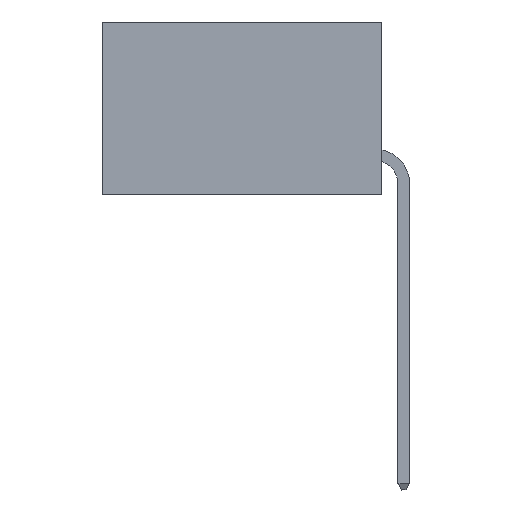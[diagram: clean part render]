
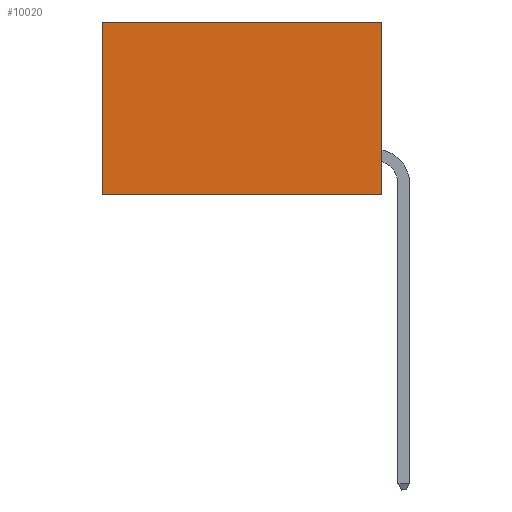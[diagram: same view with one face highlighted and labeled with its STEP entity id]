
A CAD part, left-side view. The second image highlights one B-rep face of the part: STEP entity #10020.
In plain terms, the highlighted planar face has unit normal (-1, 0, 0).
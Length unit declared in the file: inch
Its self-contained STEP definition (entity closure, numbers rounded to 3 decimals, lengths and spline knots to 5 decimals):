
#1034 = VECTOR ( 'NONE', #22122, 39.37008 ) ;
#3117 = DIRECTION ( 'NONE',  ( 1., 0., 0. ) ) ;
#3304 = DIRECTION ( 'NONE',  ( 0., 0., -1. ) ) ;
#5095 = CARTESIAN_POINT ( 'NONE',  ( 0.2875, 0., 0. ) ) ;
#5761 = EDGE_CURVE ( 'NONE', #21512, #16290, #15550, .T. ) ;
#6650 = FACE_OUTER_BOUND ( 'NONE', #12455, .T. ) ;
#6757 = AXIS2_PLACEMENT_3D ( 'NONE', #5095, #3117, #19487 ) ;
#6981 = CARTESIAN_POINT ( 'NONE',  ( 0.2875, 0., -0.37 ) ) ;
#7679 = ORIENTED_EDGE ( 'NONE', *, *, #8246, .F. ) ;
#8040 = CARTESIAN_POINT ( 'NONE',  ( 0.2875, 0., 0. ) ) ;
#8239 = PLANE ( 'NONE',  #6757 ) ;
#8246 = EDGE_CURVE ( 'NONE', #15647, #17259, #15751, .T. ) ;
#8665 = CARTESIAN_POINT ( 'NONE',  ( 0.2875, 0.6, 0. ) ) ;
#9180 = CARTESIAN_POINT ( 'NONE',  ( 0.2875, 0., 0. ) ) ;
#10020 = ADVANCED_FACE ( 'NONE', ( #6650 ), #8239, .F. ) ;
#11450 = ORIENTED_EDGE ( 'NONE', *, *, #15727, .F. ) ;
#11803 = VECTOR ( 'NONE', #3304, 39.37008 ) ;
#12327 = LINE ( 'NONE', #14745, #1034 ) ;
#12363 = VECTOR ( 'NONE', #17718, 39.37008 ) ;
#12455 = EDGE_LOOP ( 'NONE', ( #22738, #7679, #11450, #16863 ) ) ;
#12616 = LINE ( 'NONE', #19821, #11803 ) ;
#14745 = CARTESIAN_POINT ( 'NONE',  ( 0.2875, 0., 0. ) ) ;
#14821 = CARTESIAN_POINT ( 'NONE',  ( 0.2875, 0., -0.37 ) ) ;
#14979 = VECTOR ( 'NONE', #15838, 39.37008 ) ;
#15475 = EDGE_CURVE ( 'NONE', #16290, #17259, #12616, .T. ) ;
#15550 = LINE ( 'NONE', #8040, #14979 ) ;
#15647 = VERTEX_POINT ( 'NONE', #14821 ) ;
#15727 = EDGE_CURVE ( 'NONE', #21512, #15647, #12327, .T. ) ;
#15751 = LINE ( 'NONE', #6981, #12363 ) ;
#15838 = DIRECTION ( 'NONE',  ( 0., 1., 0. ) ) ;
#16290 = VERTEX_POINT ( 'NONE', #8665 ) ;
#16863 = ORIENTED_EDGE ( 'NONE', *, *, #5761, .T. ) ;
#17259 = VERTEX_POINT ( 'NONE', #22264 ) ;
#17718 = DIRECTION ( 'NONE',  ( 0., 1., 0. ) ) ;
#19487 = DIRECTION ( 'NONE',  ( 0., 0., -1. ) ) ;
#19821 = CARTESIAN_POINT ( 'NONE',  ( 0.2875, 0.6, 0. ) ) ;
#21512 = VERTEX_POINT ( 'NONE', #9180 ) ;
#22122 = DIRECTION ( 'NONE',  ( 0., 0., -1. ) ) ;
#22264 = CARTESIAN_POINT ( 'NONE',  ( 0.2875, 0.6, -0.37 ) ) ;
#22738 = ORIENTED_EDGE ( 'NONE', *, *, #15475, .T. ) ;
